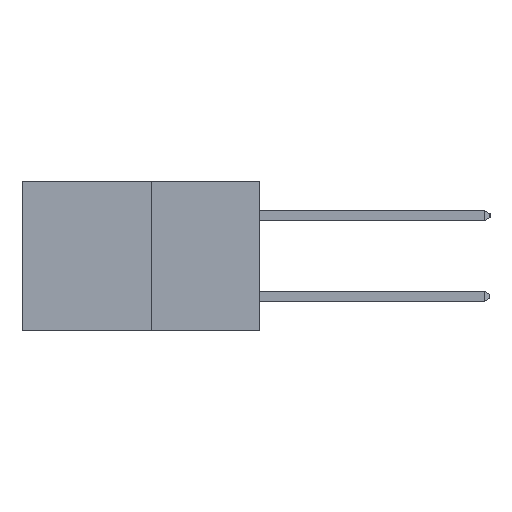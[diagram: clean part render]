
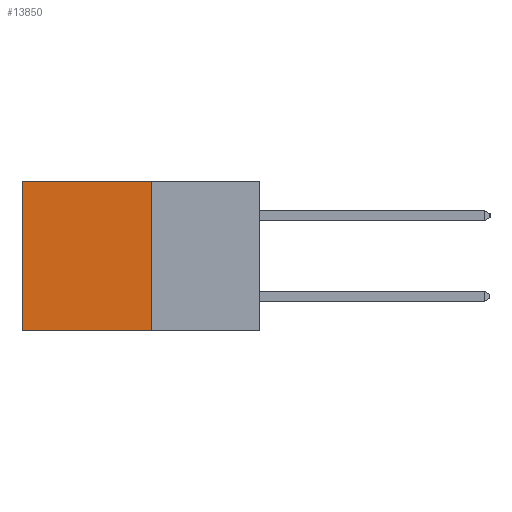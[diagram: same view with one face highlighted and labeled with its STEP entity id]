
A CAD part, left-side view. The second image highlights one B-rep face of the part: STEP entity #13850.
In plain terms, the highlighted planar face has unit normal (-1, 0, 0).
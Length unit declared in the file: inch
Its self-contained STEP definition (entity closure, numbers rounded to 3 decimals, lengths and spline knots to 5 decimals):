
#488 = VECTOR ( 'NONE', #13064, 39.37008 ) ;
#836 = FACE_OUTER_BOUND ( 'NONE', #14891, .T. ) ;
#867 = CARTESIAN_POINT ( 'NONE',  ( 0.277, 0.27, 0. ) ) ;
#938 = CARTESIAN_POINT ( 'NONE',  ( 0.277, 0.59, -0.37 ) ) ;
#1823 = CARTESIAN_POINT ( 'NONE',  ( 0.277, 0.27, -0.37 ) ) ;
#2779 = LINE ( 'NONE', #867, #16356 ) ;
#3234 = VERTEX_POINT ( 'NONE', #3733 ) ;
#3350 = DIRECTION ( 'NONE',  ( 0., 0., -1. ) ) ;
#3486 = ORIENTED_EDGE ( 'NONE', *, *, #9104, .F. ) ;
#3733 = CARTESIAN_POINT ( 'NONE',  ( 0.277, 0.27, -0.37 ) ) ;
#3930 = DIRECTION ( 'NONE',  ( 0., 0., -1. ) ) ;
#4333 = ORIENTED_EDGE ( 'NONE', *, *, #9591, .T. ) ;
#4501 = ORIENTED_EDGE ( 'NONE', *, *, #5142, .F. ) ;
#4649 = ORIENTED_EDGE ( 'NONE', *, *, #7327, .T. ) ;
#5142 = EDGE_CURVE ( 'NONE', #3234, #7167, #10683, .T. ) ;
#6062 = CARTESIAN_POINT ( 'NONE',  ( 0.277, 0.27, 0. ) ) ;
#7167 = VERTEX_POINT ( 'NONE', #10930 ) ;
#7327 = EDGE_CURVE ( 'NONE', #9689, #7167, #12430, .T. ) ;
#8602 = VECTOR ( 'NONE', #3930, 39.37008 ) ;
#9104 = EDGE_CURVE ( 'NONE', #18424, #3234, #15929, .T. ) ;
#9591 = EDGE_CURVE ( 'NONE', #18424, #9689, #2779, .T. ) ;
#9689 = VERTEX_POINT ( 'NONE', #15531 ) ;
#10683 = LINE ( 'NONE', #13309, #18229 ) ;
#10930 = CARTESIAN_POINT ( 'NONE',  ( 0.277, 0.59, -0.37 ) ) ;
#12058 = DIRECTION ( 'NONE',  ( 1., 0., 0. ) ) ;
#12430 = LINE ( 'NONE', #938, #8602 ) ;
#13064 = DIRECTION ( 'NONE',  ( 0., 0., -1. ) ) ;
#13114 = AXIS2_PLACEMENT_3D ( 'NONE', #1823, #12058, #3350 ) ;
#13283 = DIRECTION ( 'NONE',  ( 0., 1., 0. ) ) ;
#13309 = CARTESIAN_POINT ( 'NONE',  ( 0.277, 0.27, -0.37 ) ) ;
#13850 = ADVANCED_FACE ( 'NONE', ( #836 ), #17671, .F. ) ;
#14891 = EDGE_LOOP ( 'NONE', ( #4649, #4501, #3486, #4333 ) ) ;
#15531 = CARTESIAN_POINT ( 'NONE',  ( 0.277, 0.59, 0. ) ) ;
#15929 = LINE ( 'NONE', #18663, #488 ) ;
#16356 = VECTOR ( 'NONE', #18234, 39.37008 ) ;
#17671 = PLANE ( 'NONE',  #13114 ) ;
#18229 = VECTOR ( 'NONE', #13283, 39.37008 ) ;
#18234 = DIRECTION ( 'NONE',  ( 0., 1., 0. ) ) ;
#18424 = VERTEX_POINT ( 'NONE', #6062 ) ;
#18663 = CARTESIAN_POINT ( 'NONE',  ( 0.277, 0.27, -0.37 ) ) ;
